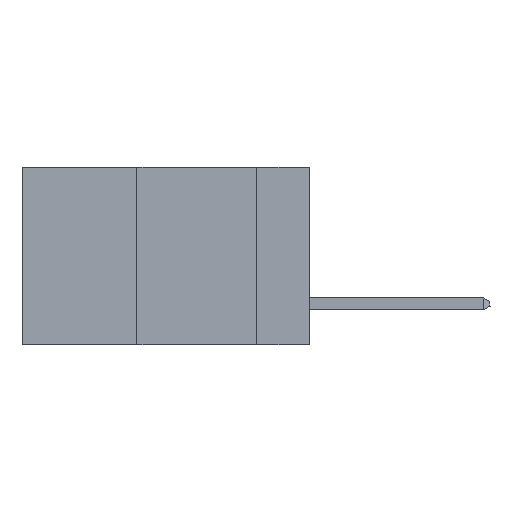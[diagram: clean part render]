
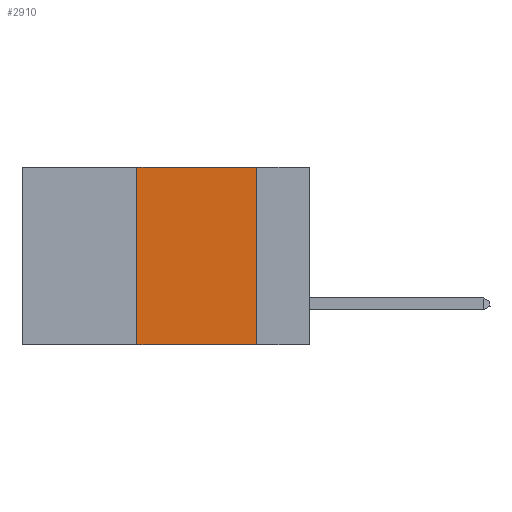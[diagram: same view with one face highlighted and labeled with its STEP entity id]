
A CAD part, left-side view. The second image highlights one B-rep face of the part: STEP entity #2910.
In plain terms, the highlighted planar face has unit normal (-1, 0, 0).
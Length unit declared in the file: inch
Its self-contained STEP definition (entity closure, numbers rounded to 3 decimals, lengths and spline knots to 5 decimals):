
#85 = CARTESIAN_POINT ( 'NONE',  ( 0., 0.11, 0. ) ) ;
#412 = AXIS2_PLACEMENT_3D ( 'NONE', #7721, #6023, #5947 ) ;
#584 = CARTESIAN_POINT ( 'NONE',  ( 0., 0.36, 0. ) ) ;
#1230 = VERTEX_POINT ( 'NONE', #584 ) ;
#1320 = FACE_OUTER_BOUND ( 'NONE', #2137, .T. ) ;
#2137 = EDGE_LOOP ( 'NONE', ( #11803, #3119, #3430, #2894 ) ) ;
#2671 = EDGE_CURVE ( 'NONE', #1230, #7498, #3609, .T. ) ;
#2867 = LINE ( 'NONE', #85, #7608 ) ;
#2894 = ORIENTED_EDGE ( 'NONE', *, *, #11190, .T. ) ;
#2910 = ADVANCED_FACE ( 'NONE', ( #1320 ), #9611, .F. ) ;
#2917 = LINE ( 'NONE', #8129, #5497 ) ;
#3119 = ORIENTED_EDGE ( 'NONE', *, *, #2671, .F. ) ;
#3430 = ORIENTED_EDGE ( 'NONE', *, *, #11855, .F. ) ;
#3609 = LINE ( 'NONE', #4623, #3910 ) ;
#3910 = VECTOR ( 'NONE', #9111, 39.37008 ) ;
#4587 = DIRECTION ( 'NONE',  ( 0., -1., 0. ) ) ;
#4623 = CARTESIAN_POINT ( 'NONE',  ( 0., 0.6, 0. ) ) ;
#5497 = VECTOR ( 'NONE', #9150, 39.37008 ) ;
#5947 = DIRECTION ( 'NONE',  ( 0., 0., -1. ) ) ;
#6023 = DIRECTION ( 'NONE',  ( 1., 0., 0. ) ) ;
#6899 = CARTESIAN_POINT ( 'NONE',  ( 0., 0.36, -0.37 ) ) ;
#7215 = VERTEX_POINT ( 'NONE', #6899 ) ;
#7356 = CARTESIAN_POINT ( 'NONE',  ( 0., 0.11, -0.37 ) ) ;
#7498 = VERTEX_POINT ( 'NONE', #11975 ) ;
#7608 = VECTOR ( 'NONE', #11181, 39.37008 ) ;
#7721 = CARTESIAN_POINT ( 'NONE',  ( 0., 0.6, 0. ) ) ;
#8129 = CARTESIAN_POINT ( 'NONE',  ( 0., 0.36, 0. ) ) ;
#8166 = LINE ( 'NONE', #11168, #10910 ) ;
#9111 = DIRECTION ( 'NONE',  ( 0., -1., 0. ) ) ;
#9150 = DIRECTION ( 'NONE',  ( 0., 0., 1. ) ) ;
#9581 = EDGE_CURVE ( 'NONE', #7498, #10058, #2867, .T. ) ;
#9611 = PLANE ( 'NONE',  #412 ) ;
#10058 = VERTEX_POINT ( 'NONE', #7356 ) ;
#10910 = VECTOR ( 'NONE', #4587, 39.37008 ) ;
#11168 = CARTESIAN_POINT ( 'NONE',  ( 0., 0.6, -0.37 ) ) ;
#11181 = DIRECTION ( 'NONE',  ( 0., 0., -1. ) ) ;
#11190 = EDGE_CURVE ( 'NONE', #7215, #10058, #8166, .T. ) ;
#11803 = ORIENTED_EDGE ( 'NONE', *, *, #9581, .F. ) ;
#11855 = EDGE_CURVE ( 'NONE', #7215, #1230, #2917, .T. ) ;
#11975 = CARTESIAN_POINT ( 'NONE',  ( 0., 0.11, 0. ) ) ;
